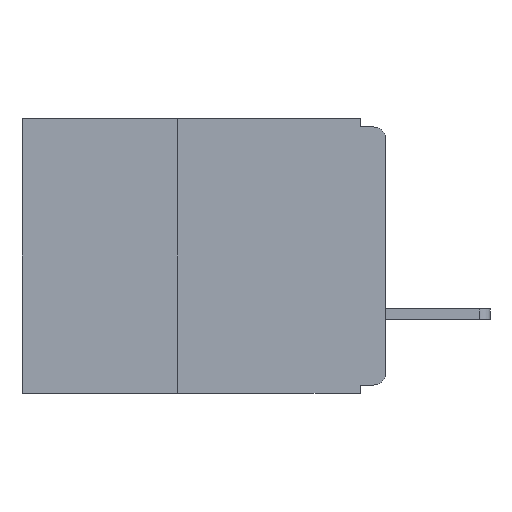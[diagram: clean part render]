
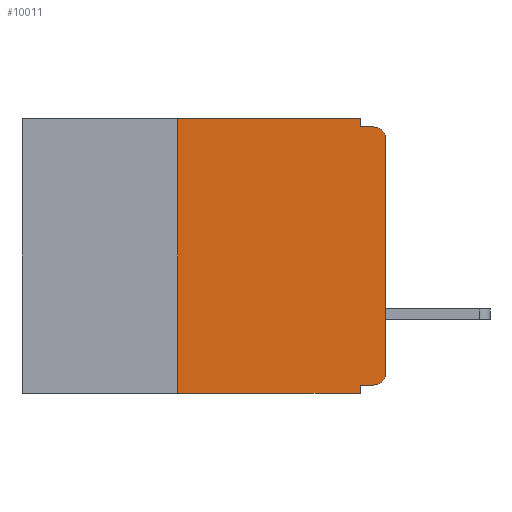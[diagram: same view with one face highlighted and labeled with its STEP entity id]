
A CAD part, left-side view. The second image highlights one B-rep face of the part: STEP entity #10011.
In plain terms, the highlighted planar face has unit normal (-1, 0, 0).
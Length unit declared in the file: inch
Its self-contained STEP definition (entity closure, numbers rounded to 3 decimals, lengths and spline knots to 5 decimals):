
#57 = CARTESIAN_POINT ( 'NONE',  ( 0., 0.031, -0.01 ) ) ;
#814 = ORIENTED_EDGE ( 'NONE', *, *, #2011, .F. ) ;
#1798 = CARTESIAN_POINT ( 'NONE',  ( 0., 0.25, 0. ) ) ;
#1846 = LINE ( 'NONE', #23500, #22350 ) ;
#2011 = EDGE_CURVE ( 'NONE', #12058, #17532, #1846, .T. ) ;
#2119 = CARTESIAN_POINT ( 'NONE',  ( 0., 0.031, -0.32 ) ) ;
#2696 = EDGE_CURVE ( 'NONE', #9512, #16477, #16564, .T. ) ;
#2823 = DIRECTION ( 'NONE',  ( -1., 0., 0. ) ) ;
#2982 = VERTEX_POINT ( 'NONE', #16886 ) ;
#3023 = LINE ( 'NONE', #11115, #13260 ) ;
#3185 = AXIS2_PLACEMENT_3D ( 'NONE', #15102, #2823, #17177 ) ;
#3398 = VECTOR ( 'NONE', #7260, 39.37008 ) ;
#3600 = DIRECTION ( 'NONE',  ( 1., 0., 0. ) ) ;
#3752 = CARTESIAN_POINT ( 'NONE',  ( 0., 0.437, -0.33 ) ) ;
#3830 = AXIS2_PLACEMENT_3D ( 'NONE', #15904, #3600, #17968 ) ;
#4574 = ORIENTED_EDGE ( 'NONE', *, *, #17192, .T. ) ;
#4641 = LINE ( 'NONE', #3752, #14962 ) ;
#5427 = CIRCLE ( 'NONE', #3185, 0.015 ) ;
#5546 = ORIENTED_EDGE ( 'NONE', *, *, #19383, .F. ) ;
#5772 = DIRECTION ( 'NONE',  ( 0., -1., 0. ) ) ;
#5862 = ORIENTED_EDGE ( 'NONE', *, *, #25721, .F. ) ;
#5998 = DIRECTION ( 'NONE',  ( 0., 0., -1. ) ) ;
#6374 = EDGE_CURVE ( 'NONE', #19869, #20978, #9458, .T. ) ;
#6402 = LINE ( 'NONE', #18351, #17379 ) ;
#6921 = LINE ( 'NONE', #25391, #11125 ) ;
#7260 = DIRECTION ( 'NONE',  ( 0., 0., -1. ) ) ;
#7834 = VERTEX_POINT ( 'NONE', #14626 ) ;
#7898 = CIRCLE ( 'NONE', #17737, 0.015 ) ;
#8241 = CARTESIAN_POINT ( 'NONE',  ( 0., 0., -0.305 ) ) ;
#8552 = CARTESIAN_POINT ( 'NONE',  ( 0., 0., -0.025 ) ) ;
#8917 = CARTESIAN_POINT ( 'NONE',  ( 0., 0.015, -0.025 ) ) ;
#9313 = CARTESIAN_POINT ( 'NONE',  ( 0., 0., -0.01 ) ) ;
#9458 = LINE ( 'NONE', #17566, #3398 ) ;
#9512 = VERTEX_POINT ( 'NONE', #14204 ) ;
#10011 = ADVANCED_FACE ( 'NONE', ( #19367 ), #26048, .F. ) ;
#10536 = DIRECTION ( 'NONE',  ( 0., 0., 1. ) ) ;
#10707 = ORIENTED_EDGE ( 'NONE', *, *, #2696, .F. ) ;
#10940 = EDGE_CURVE ( 'NONE', #16477, #2982, #6402, .T. ) ;
#10992 = DIRECTION ( 'NONE',  ( 0., 0., -1. ) ) ;
#11115 = CARTESIAN_POINT ( 'NONE',  ( 0., 0.437, 0. ) ) ;
#11125 = VECTOR ( 'NONE', #15228, 39.37008 ) ;
#11232 = EDGE_CURVE ( 'NONE', #9512, #20405, #5427, .T. ) ;
#11995 = ORIENTED_EDGE ( 'NONE', *, *, #6374, .F. ) ;
#12058 = VERTEX_POINT ( 'NONE', #13979 ) ;
#13187 = DIRECTION ( 'NONE',  ( 0., -1., 0. ) ) ;
#13260 = VECTOR ( 'NONE', #13187, 39.37008 ) ;
#13979 = CARTESIAN_POINT ( 'NONE',  ( 0., 0.25, -0.33 ) ) ;
#14204 = CARTESIAN_POINT ( 'NONE',  ( 0., 0.015, -0.32 ) ) ;
#14314 = LINE ( 'NONE', #9313, #19814 ) ;
#14538 = EDGE_CURVE ( 'NONE', #12058, #2982, #4641, .T. ) ;
#14626 = CARTESIAN_POINT ( 'NONE',  ( 0., 0.015, -0.01 ) ) ;
#14962 = VECTOR ( 'NONE', #5772, 39.37008 ) ;
#15102 = CARTESIAN_POINT ( 'NONE',  ( 0., 0.015, -0.305 ) ) ;
#15228 = DIRECTION ( 'NONE',  ( 0., 0., 1. ) ) ;
#15904 = CARTESIAN_POINT ( 'NONE',  ( 0., 0.437, 0. ) ) ;
#15926 = EDGE_LOOP ( 'NONE', ( #18425, #4574, #5862, #11995, #5546, #814, #22603, #26410, #10707, #19789 ) ) ;
#16477 = VERTEX_POINT ( 'NONE', #2119 ) ;
#16564 = LINE ( 'NONE', #23218, #21360 ) ;
#16705 = CARTESIAN_POINT ( 'NONE',  ( 0., 0.031, 0. ) ) ;
#16886 = CARTESIAN_POINT ( 'NONE',  ( 0., 0.031, -0.33 ) ) ;
#17097 = VERTEX_POINT ( 'NONE', #8552 ) ;
#17177 = DIRECTION ( 'NONE',  ( 0., 0., -1. ) ) ;
#17192 = EDGE_CURVE ( 'NONE', #17097, #7834, #7898, .T. ) ;
#17379 = VECTOR ( 'NONE', #5998, 39.37008 ) ;
#17532 = VERTEX_POINT ( 'NONE', #1798 ) ;
#17566 = CARTESIAN_POINT ( 'NONE',  ( 0., 0.031, 0. ) ) ;
#17737 = AXIS2_PLACEMENT_3D ( 'NONE', #8917, #23309, #10992 ) ;
#17968 = DIRECTION ( 'NONE',  ( 0., 0., -1. ) ) ;
#18351 = CARTESIAN_POINT ( 'NONE',  ( 0., 0.031, -0.33 ) ) ;
#18425 = ORIENTED_EDGE ( 'NONE', *, *, #25008, .T. ) ;
#19367 = FACE_OUTER_BOUND ( 'NONE', #15926, .T. ) ;
#19383 = EDGE_CURVE ( 'NONE', #17532, #19869, #3023, .T. ) ;
#19789 = ORIENTED_EDGE ( 'NONE', *, *, #11232, .T. ) ;
#19814 = VECTOR ( 'NONE', #23706, 39.37008 ) ;
#19869 = VERTEX_POINT ( 'NONE', #16705 ) ;
#20405 = VERTEX_POINT ( 'NONE', #8241 ) ;
#20978 = VERTEX_POINT ( 'NONE', #57 ) ;
#21360 = VECTOR ( 'NONE', #22281, 39.37008 ) ;
#22281 = DIRECTION ( 'NONE',  ( 0., 1., 0. ) ) ;
#22350 = VECTOR ( 'NONE', #10536, 39.37008 ) ;
#22603 = ORIENTED_EDGE ( 'NONE', *, *, #14538, .T. ) ;
#23218 = CARTESIAN_POINT ( 'NONE',  ( 0., 0., -0.32 ) ) ;
#23309 = DIRECTION ( 'NONE',  ( -1., 0., 0. ) ) ;
#23500 = CARTESIAN_POINT ( 'NONE',  ( 0., 0.25, -0.33 ) ) ;
#23706 = DIRECTION ( 'NONE',  ( 0., -1., 0. ) ) ;
#25008 = EDGE_CURVE ( 'NONE', #20405, #17097, #6921, .T. ) ;
#25391 = CARTESIAN_POINT ( 'NONE',  ( 0., 0., 0. ) ) ;
#25721 = EDGE_CURVE ( 'NONE', #20978, #7834, #14314, .T. ) ;
#26048 = PLANE ( 'NONE',  #3830 ) ;
#26410 = ORIENTED_EDGE ( 'NONE', *, *, #10940, .F. ) ;
